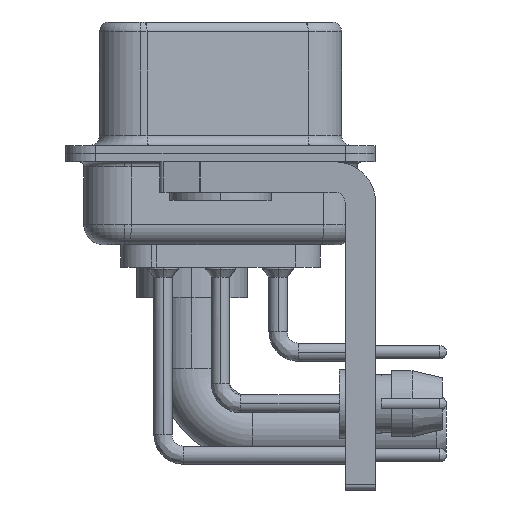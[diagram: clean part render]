
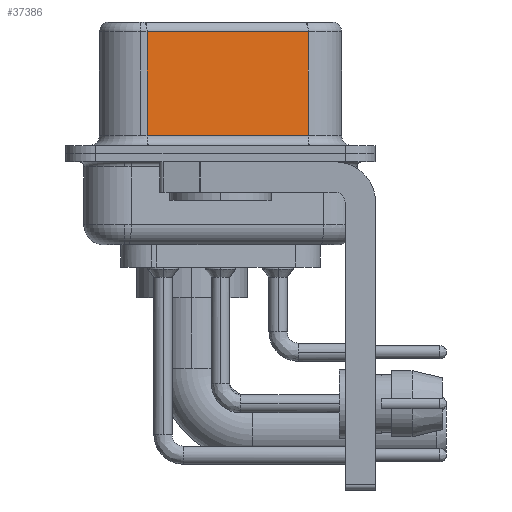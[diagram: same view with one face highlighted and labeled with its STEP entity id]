
A CAD part, left-side view. The second image highlights one B-rep face of the part: STEP entity #37386.
In plain terms, the highlighted planar face has unit normal (-0.985, -0.174, 0).
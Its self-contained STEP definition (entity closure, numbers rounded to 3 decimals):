
#693 = ORIENTED_EDGE ( 'NONE', *, *, #38343, .T. ) ;
#889 = VERTEX_POINT ( 'NONE', #20759 ) ;
#1675 = CARTESIAN_POINT ( 'NONE',  ( 3.73, 3.628, 0.9 ) ) ;
#1896 = EDGE_CURVE ( 'NONE', #15754, #21220, #37065, .T. ) ;
#2996 = ORIENTED_EDGE ( 'NONE', *, *, #1896, .F. ) ;
#4672 = EDGE_CURVE ( 'NONE', #14598, #21220, #29312, .T. ) ;
#7360 = CARTESIAN_POINT ( 'NONE',  ( 5.132, -4.322, 6.52 ) ) ;
#14598 = VERTEX_POINT ( 'NONE', #1675 ) ;
#14737 = CARTESIAN_POINT ( 'NONE',  ( 5.132, -4.322, 6.02 ) ) ;
#15433 = CARTESIAN_POINT ( 'NONE',  ( 5.132, -4.322, 6.02 ) ) ;
#15754 = VERTEX_POINT ( 'NONE', #15433 ) ;
#15799 = CARTESIAN_POINT ( 'NONE',  ( 5.132, -4.322, 6.52 ) ) ;
#16329 = AXIS2_PLACEMENT_3D ( 'NONE', #15799, #27714, #31041 ) ;
#16364 = EDGE_LOOP ( 'NONE', ( #2996, #37939, #693, #36445 ) ) ;
#16715 = CARTESIAN_POINT ( 'NONE',  ( 3.73, 3.628, 6.52 ) ) ;
#16814 = DIRECTION ( 'NONE',  ( 0.174, -0.985, 0. ) ) ;
#18462 = VECTOR ( 'NONE', #33942, 1000. ) ;
#19822 = DIRECTION ( 'NONE',  ( -0.174, 0.985, 0. ) ) ;
#20759 = CARTESIAN_POINT ( 'NONE',  ( 3.73, 3.628, 6.02 ) ) ;
#21220 = VERTEX_POINT ( 'NONE', #28896 ) ;
#22874 = CARTESIAN_POINT ( 'NONE',  ( 5.132, -4.322, 0.9 ) ) ;
#26350 = VECTOR ( 'NONE', #34681, 1000. ) ;
#26454 = LINE ( 'NONE', #14737, #32772 ) ;
#27714 = DIRECTION ( 'NONE',  ( 0.985, 0.174, 0. ) ) ;
#28455 = LINE ( 'NONE', #16715, #26350 ) ;
#28896 = CARTESIAN_POINT ( 'NONE',  ( 5.132, -4.322, 0.9 ) ) ;
#29312 = LINE ( 'NONE', #22874, #37324 ) ;
#30974 = EDGE_CURVE ( 'NONE', #15754, #889, #26454, .T. ) ;
#31041 = DIRECTION ( 'NONE',  ( -0.174, 0.985, 0. ) ) ;
#31221 = PLANE ( 'NONE',  #16329 ) ;
#32772 = VECTOR ( 'NONE', #19822, 1000. ) ;
#33942 = DIRECTION ( 'NONE',  ( 0., 0., -1. ) ) ;
#33963 = FACE_OUTER_BOUND ( 'NONE', #16364, .T. ) ;
#34681 = DIRECTION ( 'NONE',  ( 0., 0., -1. ) ) ;
#36445 = ORIENTED_EDGE ( 'NONE', *, *, #4672, .T. ) ;
#37065 = LINE ( 'NONE', #7360, #18462 ) ;
#37324 = VECTOR ( 'NONE', #16814, 1000. ) ;
#37386 = ADVANCED_FACE ( 'NONE', ( #33963 ), #31221, .F. ) ;
#37939 = ORIENTED_EDGE ( 'NONE', *, *, #30974, .T. ) ;
#38343 = EDGE_CURVE ( 'NONE', #889, #14598, #28455, .T. ) ;
